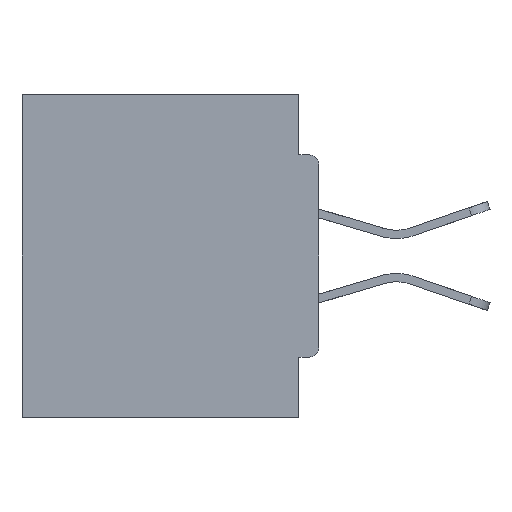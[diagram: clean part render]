
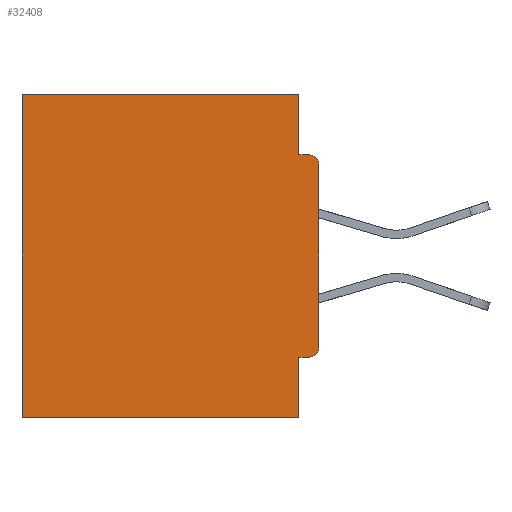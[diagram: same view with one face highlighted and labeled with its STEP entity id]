
A CAD part, left-side view. The second image highlights one B-rep face of the part: STEP entity #32408.
In plain terms, the highlighted planar face has unit normal (-1, 0, 0).
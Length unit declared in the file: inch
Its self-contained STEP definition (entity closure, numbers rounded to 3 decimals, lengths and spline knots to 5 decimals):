
#333 = EDGE_CURVE ( 'NONE', #25409, #11015, #24171, .T. ) ;
#391 = EDGE_LOOP ( 'NONE', ( #26444, #12296, #2677, #11275, #10600, #30469, #33084, #1401, #3112, #7462 ) ) ;
#845 = DIRECTION ( 'NONE',  ( 0., 0., -1. ) ) ;
#1058 = CIRCLE ( 'NONE', #31797, 0.015 ) ;
#1098 = VERTEX_POINT ( 'NONE', #26740 ) ;
#1401 = ORIENTED_EDGE ( 'NONE', *, *, #333, .F. ) ;
#1575 = CARTESIAN_POINT ( 'NONE',  ( 0.298, 0.015, -0.0935 ) ) ;
#1720 = VECTOR ( 'NONE', #18431, 39.37008 ) ;
#1766 = VERTEX_POINT ( 'NONE', #29282 ) ;
#2535 = VERTEX_POINT ( 'NONE', #14273 ) ;
#2677 = ORIENTED_EDGE ( 'NONE', *, *, #30280, .F. ) ;
#2830 = VERTEX_POINT ( 'NONE', #11134 ) ;
#2848 = EDGE_CURVE ( 'NONE', #2830, #30738, #7486, .T. ) ;
#3112 = ORIENTED_EDGE ( 'NONE', *, *, #16987, .T. ) ;
#3974 = DIRECTION ( 'NONE',  ( 0., 0., -1. ) ) ;
#5283 = CARTESIAN_POINT ( 'NONE',  ( 0.298, 0., 0. ) ) ;
#5512 = VECTOR ( 'NONE', #29068, 39.37008 ) ;
#6356 = FACE_OUTER_BOUND ( 'NONE', #391, .T. ) ;
#7220 = CARTESIAN_POINT ( 'NONE',  ( 0.298, 0., -0.4065 ) ) ;
#7462 = ORIENTED_EDGE ( 'NONE', *, *, #21739, .F. ) ;
#7486 = LINE ( 'NONE', #11024, #5512 ) ;
#8098 = EDGE_CURVE ( 'NONE', #1098, #2535, #11125, .T. ) ;
#8816 = DIRECTION ( 'NONE',  ( 0., 0., -1. ) ) ;
#9083 = CARTESIAN_POINT ( 'NONE',  ( 0.298, 0.031, -0.0935 ) ) ;
#9405 = CARTESIAN_POINT ( 'NONE',  ( 0.298, 0.031, -0.4065 ) ) ;
#9503 = EDGE_CURVE ( 'NONE', #30738, #2535, #11002, .T. ) ;
#10600 = ORIENTED_EDGE ( 'NONE', *, *, #9503, .T. ) ;
#11002 = LINE ( 'NONE', #16754, #13825 ) ;
#11015 = VERTEX_POINT ( 'NONE', #9405 ) ;
#11024 = CARTESIAN_POINT ( 'NONE',  ( 0.298, 0., 0. ) ) ;
#11125 = LINE ( 'NONE', #33003, #30068 ) ;
#11134 = CARTESIAN_POINT ( 'NONE',  ( 0.298, 0.031, 0. ) ) ;
#11275 = ORIENTED_EDGE ( 'NONE', *, *, #2848, .T. ) ;
#11490 = LINE ( 'NONE', #30017, #23206 ) ;
#12296 = ORIENTED_EDGE ( 'NONE', *, *, #16784, .F. ) ;
#12403 = DIRECTION ( 'NONE',  ( 0., 1., 0. ) ) ;
#13699 = AXIS2_PLACEMENT_3D ( 'NONE', #17049, #19550, #22213 ) ;
#13825 = VECTOR ( 'NONE', #24406, 39.37008 ) ;
#14273 = CARTESIAN_POINT ( 'NONE',  ( 0.298, 0.46, -0.5 ) ) ;
#14479 = DIRECTION ( 'NONE',  ( 0., 0., -1. ) ) ;
#16754 = CARTESIAN_POINT ( 'NONE',  ( 0.298, 0.46, 0. ) ) ;
#16784 = EDGE_CURVE ( 'NONE', #31000, #29957, #11490, .T. ) ;
#16801 = AXIS2_PLACEMENT_3D ( 'NONE', #22329, #32469, #14479 ) ;
#16987 = EDGE_CURVE ( 'NONE', #25409, #26250, #1058, .T. ) ;
#17049 = CARTESIAN_POINT ( 'NONE',  ( 0.298, 0., 0. ) ) ;
#17301 = VECTOR ( 'NONE', #12403, 39.37008 ) ;
#17993 = EDGE_CURVE ( 'NONE', #11015, #1098, #30532, .T. ) ;
#18431 = DIRECTION ( 'NONE',  ( 0., 0., -1. ) ) ;
#18661 = VECTOR ( 'NONE', #845, 39.37008 ) ;
#19043 = LINE ( 'NONE', #5283, #18661 ) ;
#19550 = DIRECTION ( 'NONE',  ( 1., 0., 0. ) ) ;
#20782 = PLANE ( 'NONE',  #13699 ) ;
#20896 = CARTESIAN_POINT ( 'NONE',  ( 0.298, 0.031, -0.5 ) ) ;
#21739 = EDGE_CURVE ( 'NONE', #1766, #26250, #19043, .T. ) ;
#21874 = CARTESIAN_POINT ( 'NONE',  ( 0.298, 0.015, -0.3915 ) ) ;
#22213 = DIRECTION ( 'NONE',  ( 0., 0., -1. ) ) ;
#22225 = LINE ( 'NONE', #20896, #1720 ) ;
#22229 = DIRECTION ( 'NONE',  ( 0., -1., 0. ) ) ;
#22329 = CARTESIAN_POINT ( 'NONE',  ( 0.298, 0.015, -0.1085 ) ) ;
#23192 = CARTESIAN_POINT ( 'NONE',  ( 0.298, 0.46, 0. ) ) ;
#23206 = VECTOR ( 'NONE', #22229, 39.37008 ) ;
#23587 = DIRECTION ( 'NONE',  ( 0., 1., 0. ) ) ;
#24022 = CARTESIAN_POINT ( 'NONE',  ( 0.298, 0., -0.3915 ) ) ;
#24171 = LINE ( 'NONE', #7220, #17301 ) ;
#24359 = CARTESIAN_POINT ( 'NONE',  ( 0.298, 0.031, -0.5 ) ) ;
#24406 = DIRECTION ( 'NONE',  ( 0., 0., -1. ) ) ;
#24917 = VECTOR ( 'NONE', #8816, 39.37008 ) ;
#25409 = VERTEX_POINT ( 'NONE', #32545 ) ;
#25895 = EDGE_CURVE ( 'NONE', #1766, #29957, #27453, .T. ) ;
#26250 = VERTEX_POINT ( 'NONE', #24022 ) ;
#26444 = ORIENTED_EDGE ( 'NONE', *, *, #25895, .T. ) ;
#26740 = CARTESIAN_POINT ( 'NONE',  ( 0.298, 0.031, -0.5 ) ) ;
#27453 = CIRCLE ( 'NONE', #16801, 0.015 ) ;
#29068 = DIRECTION ( 'NONE',  ( 0., 1., 0. ) ) ;
#29282 = CARTESIAN_POINT ( 'NONE',  ( 0.298, 0., -0.1085 ) ) ;
#29957 = VERTEX_POINT ( 'NONE', #1575 ) ;
#30017 = CARTESIAN_POINT ( 'NONE',  ( 0.298, 0., -0.0935 ) ) ;
#30068 = VECTOR ( 'NONE', #23587, 39.37008 ) ;
#30280 = EDGE_CURVE ( 'NONE', #2830, #31000, #22225, .T. ) ;
#30469 = ORIENTED_EDGE ( 'NONE', *, *, #8098, .F. ) ;
#30532 = LINE ( 'NONE', #24359, #24917 ) ;
#30738 = VERTEX_POINT ( 'NONE', #23192 ) ;
#31000 = VERTEX_POINT ( 'NONE', #9083 ) ;
#31797 = AXIS2_PLACEMENT_3D ( 'NONE', #21874, #32130, #3974 ) ;
#32130 = DIRECTION ( 'NONE',  ( -1., 0., 0. ) ) ;
#32408 = ADVANCED_FACE ( 'NONE', ( #6356 ), #20782, .F. ) ;
#32469 = DIRECTION ( 'NONE',  ( -1., 0., 0. ) ) ;
#32545 = CARTESIAN_POINT ( 'NONE',  ( 0.298, 0.015, -0.4065 ) ) ;
#33003 = CARTESIAN_POINT ( 'NONE',  ( 0.298, 0., -0.5 ) ) ;
#33084 = ORIENTED_EDGE ( 'NONE', *, *, #17993, .F. ) ;
